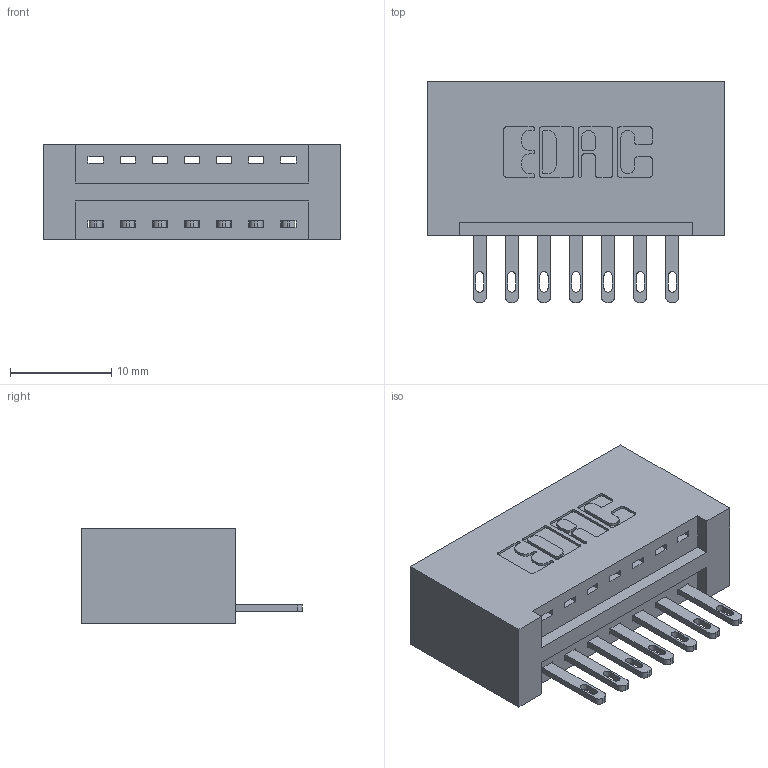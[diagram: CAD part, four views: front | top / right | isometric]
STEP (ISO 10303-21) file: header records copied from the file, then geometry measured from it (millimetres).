
FILE_DESCRIPTION (( 'STEP AP203' ), '1' );
FILE_NAME ('346-007-500-101.STEP', '2022-05-04T19:20:00', ( '' ), ( '' ), 'SwSTEP 2.0', 'SolidWorks 2020', '' );
FILE_SCHEMA (( 'CONFIG_CONTROL_DESIGN' ));
Length unit declared in the file: inch
Products named in the file (3): 345-292-001_345-293-100; 346-007-500-101; 346 Part_No Mounting Lugs
Assembly tree (8 placements, depth 2):
  346-007-500-101
    346 Part_No Mounting Lugs
    345-292-001_345-293-100  x7
Bounding box: 29.46 x 21.84 x 9.4 mm (x, y, z)
Volume: 3133 mm3; surface area: 3629.5 mm2
Topology: 8 solids, 8 shells, 492 faces, 1481 edges, 986 vertices
Faces by surface type: plane 310, cylinder 182
Entity records: 8709 total; most frequent: CARTESIAN_POINT 1509, ORIENTED_EDGE 1450, DIRECTION 1371, EDGE_CURVE 725, VECTOR 569, LINE 569, VERTEX_POINT 482, AXIS2_PLACEMENT_3D 401
